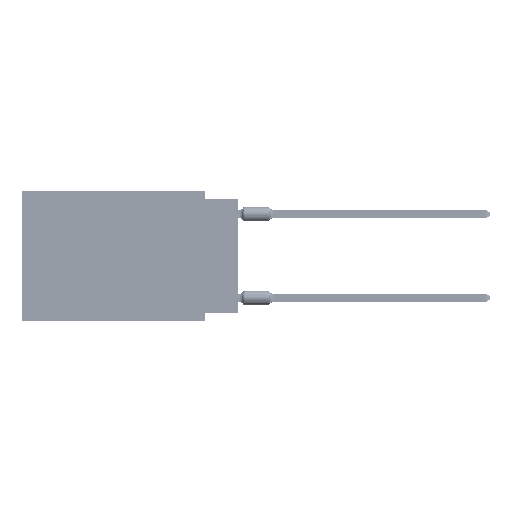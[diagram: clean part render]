
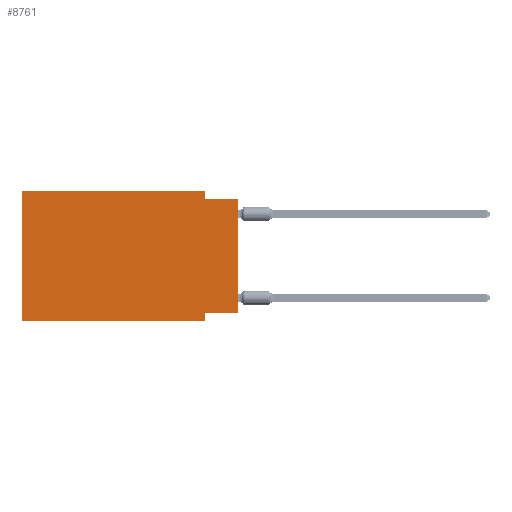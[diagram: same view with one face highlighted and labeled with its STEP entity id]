
A CAD part, left-side view. The second image highlights one B-rep face of the part: STEP entity #8761.
In plain terms, the highlighted planar face has unit normal (-1, 0, 0).
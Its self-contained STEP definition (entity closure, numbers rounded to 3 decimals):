
#1533 = DIRECTION ( 'NONE',  ( 0., 0., -1. ) ) ;
#1903 = EDGE_CURVE ( 'NONE', #11699, #64545, #10256, .T. ) ;
#3771 = VERTEX_POINT ( 'NONE', #36355 ) ;
#5587 = DIRECTION ( 'NONE',  ( 1., 0., 0. ) ) ;
#6264 = DIRECTION ( 'NONE',  ( 0., -1., 0. ) ) ;
#8761 = ADVANCED_FACE ( 'NONE', ( #62080 ), #33831, .F. ) ;
#9369 = DIRECTION ( 'NONE',  ( 0., 0., 1. ) ) ;
#9692 = CARTESIAN_POINT ( 'NONE',  ( 0., 0., 0. ) ) ;
#9766 = EDGE_CURVE ( 'NONE', #37859, #19852, #27675, .T. ) ;
#10256 = LINE ( 'NONE', #50843, #29851 ) ;
#10566 = VECTOR ( 'NONE', #76029, 1000. ) ;
#11699 = VERTEX_POINT ( 'NONE', #24745 ) ;
#11725 = EDGE_CURVE ( 'NONE', #11699, #3771, #46172, .T. ) ;
#15545 = CARTESIAN_POINT ( 'NONE',  ( 0., 16.383, 0. ) ) ;
#16969 = LINE ( 'NONE', #9692, #32222 ) ;
#18006 = EDGE_CURVE ( 'NONE', #38264, #3771, #47588, .T. ) ;
#18236 = ORIENTED_EDGE ( 'NONE', *, *, #89052, .T. ) ;
#19852 = VERTEX_POINT ( 'NONE', #81253 ) ;
#20447 = CARTESIAN_POINT ( 'NONE',  ( 0., 16.383, 0. ) ) ;
#21946 = EDGE_LOOP ( 'NONE', ( #18236, #36781, #40211, #33670, #68537, #30915, #77188, #78208 ) ) ;
#22014 = DIRECTION ( 'NONE',  ( 0., 1., 0. ) ) ;
#22462 = LINE ( 'NONE', #57108, #75875 ) ;
#22855 = EDGE_CURVE ( 'NONE', #34594, #38264, #63029, .T. ) ;
#23897 = CARTESIAN_POINT ( 'NONE',  ( 0., 0., -9.271 ) ) ;
#24745 = CARTESIAN_POINT ( 'NONE',  ( 0., 16.383, -9.906 ) ) ;
#27271 = CARTESIAN_POINT ( 'NONE',  ( 0., 2.54, -9.271 ) ) ;
#27675 = LINE ( 'NONE', #49545, #56709 ) ;
#29851 = VECTOR ( 'NONE', #9369, 1000. ) ;
#30915 = ORIENTED_EDGE ( 'NONE', *, *, #11725, .T. ) ;
#32222 = VECTOR ( 'NONE', #37922, 1000. ) ;
#32934 = CARTESIAN_POINT ( 'NONE',  ( 0., 2.54, 0. ) ) ;
#33670 = ORIENTED_EDGE ( 'NONE', *, *, #89761, .F. ) ;
#33831 = PLANE ( 'NONE',  #43578 ) ;
#34357 = CARTESIAN_POINT ( 'NONE',  ( 0., 2.54, -9.906 ) ) ;
#34594 = VERTEX_POINT ( 'NONE', #23897 ) ;
#36236 = VECTOR ( 'NONE', #22014, 1000. ) ;
#36355 = CARTESIAN_POINT ( 'NONE',  ( 0., 2.54, -9.906 ) ) ;
#36781 = ORIENTED_EDGE ( 'NONE', *, *, #9766, .F. ) ;
#37859 = VERTEX_POINT ( 'NONE', #40155 ) ;
#37922 = DIRECTION ( 'NONE',  ( 0., 0., 1. ) ) ;
#38264 = VERTEX_POINT ( 'NONE', #27271 ) ;
#40155 = CARTESIAN_POINT ( 'NONE',  ( 0., 2.54, -0.635 ) ) ;
#40211 = ORIENTED_EDGE ( 'NONE', *, *, #88802, .F. ) ;
#43578 = AXIS2_PLACEMENT_3D ( 'NONE', #89864, #5587, #61616 ) ;
#46172 = LINE ( 'NONE', #73048, #84411 ) ;
#47588 = LINE ( 'NONE', #34357, #66299 ) ;
#49545 = CARTESIAN_POINT ( 'NONE',  ( 0., 0., -0.635 ) ) ;
#50843 = CARTESIAN_POINT ( 'NONE',  ( 0., 16.383, 0. ) ) ;
#55088 = LINE ( 'NONE', #20447, #10566 ) ;
#56709 = VECTOR ( 'NONE', #6264, 1000. ) ;
#57108 = CARTESIAN_POINT ( 'NONE',  ( 0., 2.54, 0. ) ) ;
#61616 = DIRECTION ( 'NONE',  ( 0., 0., -1. ) ) ;
#62080 = FACE_OUTER_BOUND ( 'NONE', #21946, .T. ) ;
#62577 = CARTESIAN_POINT ( 'NONE',  ( 0., 0., -9.271 ) ) ;
#63029 = LINE ( 'NONE', #62577, #36236 ) ;
#64545 = VERTEX_POINT ( 'NONE', #15545 ) ;
#66299 = VECTOR ( 'NONE', #83097, 1000. ) ;
#68195 = VERTEX_POINT ( 'NONE', #32934 ) ;
#68537 = ORIENTED_EDGE ( 'NONE', *, *, #1903, .F. ) ;
#73048 = CARTESIAN_POINT ( 'NONE',  ( 0., 16.383, -9.906 ) ) ;
#75875 = VECTOR ( 'NONE', #1533, 1000. ) ;
#76029 = DIRECTION ( 'NONE',  ( 0., -1., 0. ) ) ;
#77188 = ORIENTED_EDGE ( 'NONE', *, *, #18006, .F. ) ;
#78208 = ORIENTED_EDGE ( 'NONE', *, *, #22855, .F. ) ;
#81253 = CARTESIAN_POINT ( 'NONE',  ( 0., 0., -0.635 ) ) ;
#83097 = DIRECTION ( 'NONE',  ( 0., 0., -1. ) ) ;
#84411 = VECTOR ( 'NONE', #87611, 1000. ) ;
#87611 = DIRECTION ( 'NONE',  ( 0., -1., 0. ) ) ;
#88802 = EDGE_CURVE ( 'NONE', #68195, #37859, #22462, .T. ) ;
#89052 = EDGE_CURVE ( 'NONE', #34594, #19852, #16969, .T. ) ;
#89761 = EDGE_CURVE ( 'NONE', #64545, #68195, #55088, .T. ) ;
#89864 = CARTESIAN_POINT ( 'NONE',  ( 0., 16.383, 0. ) ) ;
